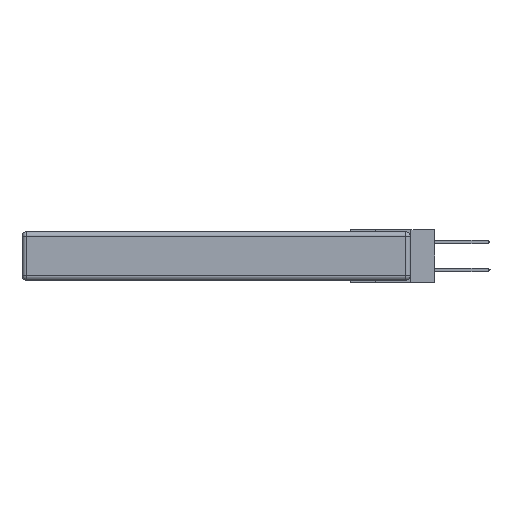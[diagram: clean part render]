
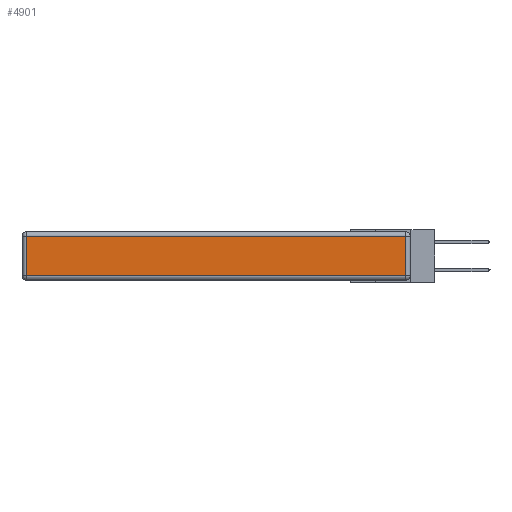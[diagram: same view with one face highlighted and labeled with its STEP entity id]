
A CAD part, left-side view. The second image highlights one B-rep face of the part: STEP entity #4901.
In plain terms, the highlighted planar face has unit normal (-1, 0, 0).
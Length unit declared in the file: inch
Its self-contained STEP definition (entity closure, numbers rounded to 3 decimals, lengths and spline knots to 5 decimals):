
#127 = CARTESIAN_POINT ( 'NONE',  ( 0., 0.03, -0.03 ) ) ;
#169 = VECTOR ( 'NONE', #12547, 39.37008 ) ;
#358 = CARTESIAN_POINT ( 'NONE',  ( 0., 2.72, -0.03 ) ) ;
#1422 = ORIENTED_EDGE ( 'NONE', *, *, #4247, .T. ) ;
#1671 = DIRECTION ( 'NONE',  ( 0., 1., 0. ) ) ;
#1814 = VECTOR ( 'NONE', #1671, 39.37008 ) ;
#2049 = VECTOR ( 'NONE', #4618, 39.37008 ) ;
#3133 = VERTEX_POINT ( 'NONE', #358 ) ;
#3186 = LINE ( 'NONE', #6863, #1814 ) ;
#3446 = DIRECTION ( 'NONE',  ( -1., 0., 0. ) ) ;
#4247 = EDGE_CURVE ( 'NONE', #5718, #3133, #3186, .T. ) ;
#4618 = DIRECTION ( 'NONE',  ( 0., 0., -1. ) ) ;
#4757 = EDGE_CURVE ( 'NONE', #7734, #18275, #9458, .T. ) ;
#4901 = ADVANCED_FACE ( 'NONE', ( #12727 ), #14532, .T. ) ;
#5622 = EDGE_CURVE ( 'NONE', #18275, #5718, #19513, .T. ) ;
#5718 = VERTEX_POINT ( 'NONE', #127 ) ;
#6863 = CARTESIAN_POINT ( 'NONE',  ( 0., 2.75, -0.03 ) ) ;
#6870 = CARTESIAN_POINT ( 'NONE',  ( 0., 0., -0.343 ) ) ;
#7734 = VERTEX_POINT ( 'NONE', #15603 ) ;
#8067 = CARTESIAN_POINT ( 'NONE',  ( 0., 2.72, -0.343 ) ) ;
#9458 = LINE ( 'NONE', #17811, #169 ) ;
#9670 = VECTOR ( 'NONE', #14772, 39.37008 ) ;
#9675 = ORIENTED_EDGE ( 'NONE', *, *, #13043, .T. ) ;
#10316 = EDGE_LOOP ( 'NONE', ( #11785, #18394, #1422, #9675 ) ) ;
#11785 = ORIENTED_EDGE ( 'NONE', *, *, #4757, .T. ) ;
#12547 = DIRECTION ( 'NONE',  ( 0., -1., 0. ) ) ;
#12727 = FACE_OUTER_BOUND ( 'NONE', #10316, .T. ) ;
#13043 = EDGE_CURVE ( 'NONE', #3133, #7734, #16823, .T. ) ;
#14164 = CARTESIAN_POINT ( 'NONE',  ( 0., 0.03, -0.343 ) ) ;
#14532 = PLANE ( 'NONE',  #16589 ) ;
#14772 = DIRECTION ( 'NONE',  ( 0., 0., 1. ) ) ;
#15603 = CARTESIAN_POINT ( 'NONE',  ( 0., 2.72, -0.313 ) ) ;
#16589 = AXIS2_PLACEMENT_3D ( 'NONE', #6870, #3446, #21009 ) ;
#16823 = LINE ( 'NONE', #8067, #2049 ) ;
#17811 = CARTESIAN_POINT ( 'NONE',  ( 0., 0., -0.313 ) ) ;
#18275 = VERTEX_POINT ( 'NONE', #21091 ) ;
#18394 = ORIENTED_EDGE ( 'NONE', *, *, #5622, .T. ) ;
#19513 = LINE ( 'NONE', #14164, #9670 ) ;
#21009 = DIRECTION ( 'NONE',  ( 0., 0., 1. ) ) ;
#21091 = CARTESIAN_POINT ( 'NONE',  ( 0., 0.03, -0.313 ) ) ;
